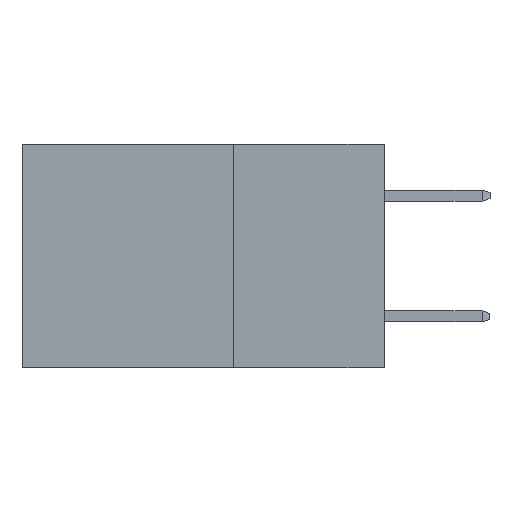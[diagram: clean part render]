
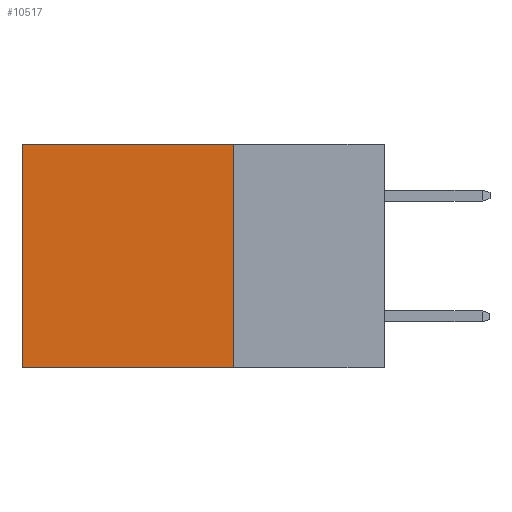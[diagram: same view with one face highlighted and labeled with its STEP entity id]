
A CAD part, left-side view. The second image highlights one B-rep face of the part: STEP entity #10517.
In plain terms, the highlighted planar face has unit normal (-1, 0, 0).
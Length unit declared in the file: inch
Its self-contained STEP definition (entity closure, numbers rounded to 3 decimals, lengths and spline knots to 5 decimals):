
#980 = CARTESIAN_POINT ( 'NONE',  ( 0.298, 0.25, 0. ) ) ;
#1482 = ORIENTED_EDGE ( 'NONE', *, *, #4300, .T. ) ;
#1537 = ORIENTED_EDGE ( 'NONE', *, *, #7013, .F. ) ;
#1615 = ORIENTED_EDGE ( 'NONE', *, *, #14736, .F. ) ;
#1626 = ORIENTED_EDGE ( 'NONE', *, *, #16345, .T. ) ;
#3103 = DIRECTION ( 'NONE',  ( 0., 1., 0. ) ) ;
#3126 = CARTESIAN_POINT ( 'NONE',  ( 0.298, 0.25, 0. ) ) ;
#4136 = DIRECTION ( 'NONE',  ( 0., 0., -1. ) ) ;
#4234 = CARTESIAN_POINT ( 'NONE',  ( 0.298, 0.25, -0.37 ) ) ;
#4300 = EDGE_CURVE ( 'NONE', #10279, #14835, #11772, .T. ) ;
#5294 = CARTESIAN_POINT ( 'NONE',  ( 0.298, 0.25, 0. ) ) ;
#5475 = VERTEX_POINT ( 'NONE', #4234 ) ;
#5719 = CARTESIAN_POINT ( 'NONE',  ( 0.298, 0.25, 0. ) ) ;
#7013 = EDGE_CURVE ( 'NONE', #5475, #14835, #7552, .T. ) ;
#7502 = CARTESIAN_POINT ( 'NONE',  ( 0.298, 0.6, 0. ) ) ;
#7552 = LINE ( 'NONE', #12798, #13825 ) ;
#7944 = DIRECTION ( 'NONE',  ( 0., 0., -1. ) ) ;
#8050 = FACE_OUTER_BOUND ( 'NONE', #12536, .T. ) ;
#8414 = VECTOR ( 'NONE', #4136, 39.37008 ) ;
#10279 = VERTEX_POINT ( 'NONE', #7502 ) ;
#10320 = CARTESIAN_POINT ( 'NONE',  ( 0.298, 0.6, 0. ) ) ;
#10385 = AXIS2_PLACEMENT_3D ( 'NONE', #5294, #15413, #7944 ) ;
#10517 = ADVANCED_FACE ( 'NONE', ( #8050 ), #12917, .F. ) ;
#11376 = DIRECTION ( 'NONE',  ( 0., 1., 0. ) ) ;
#11772 = LINE ( 'NONE', #10320, #8414 ) ;
#12301 = LINE ( 'NONE', #3126, #15554 ) ;
#12536 = EDGE_LOOP ( 'NONE', ( #1482, #1537, #1615, #1626 ) ) ;
#12798 = CARTESIAN_POINT ( 'NONE',  ( 0.298, 0.25, -0.37 ) ) ;
#12917 = PLANE ( 'NONE',  #10385 ) ;
#13226 = VECTOR ( 'NONE', #3103, 39.37008 ) ;
#13403 = DIRECTION ( 'NONE',  ( 0., 0., -1. ) ) ;
#13614 = LINE ( 'NONE', #5719, #13226 ) ;
#13647 = VERTEX_POINT ( 'NONE', #980 ) ;
#13825 = VECTOR ( 'NONE', #11376, 39.37008 ) ;
#14698 = CARTESIAN_POINT ( 'NONE',  ( 0.298, 0.6, -0.37 ) ) ;
#14736 = EDGE_CURVE ( 'NONE', #13647, #5475, #12301, .T. ) ;
#14835 = VERTEX_POINT ( 'NONE', #14698 ) ;
#15413 = DIRECTION ( 'NONE',  ( 1., 0., 0. ) ) ;
#15554 = VECTOR ( 'NONE', #13403, 39.37008 ) ;
#16345 = EDGE_CURVE ( 'NONE', #13647, #10279, #13614, .T. ) ;
